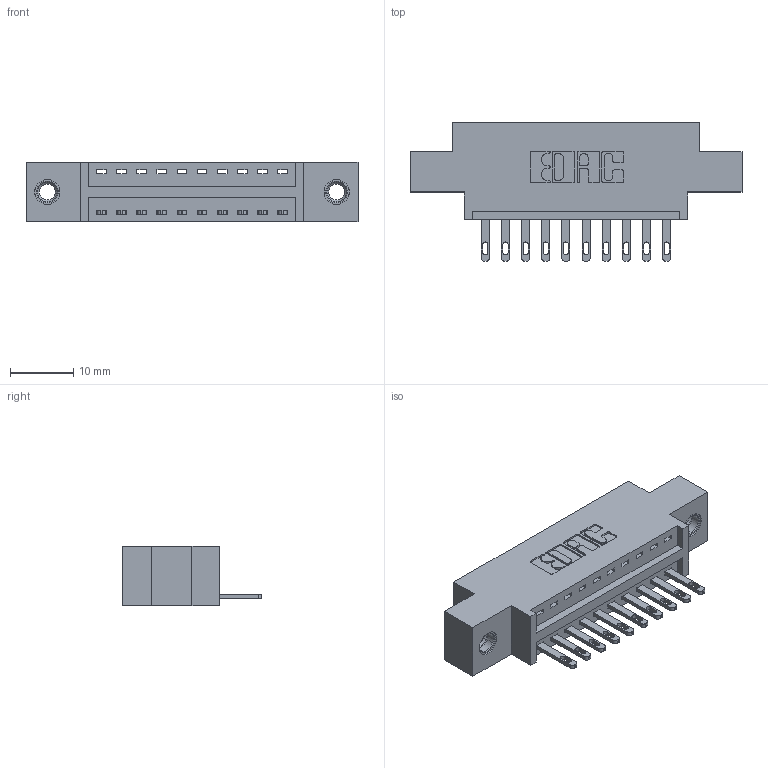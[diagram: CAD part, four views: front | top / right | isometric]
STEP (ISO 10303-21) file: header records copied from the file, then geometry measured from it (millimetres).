
FILE_DESCRIPTION (( 'STEP AP203' ), '1' );
FILE_NAME ('896-010-500-607.STEP', '2021-07-27T14:25:12', ( '' ), ( '' ), 'SwSTEP 2.0', 'SolidWorks 2020', '' );
FILE_SCHEMA (( 'CONFIG_CONTROL_DESIGN' ));
Length unit declared in the file: inch
Products named in the file (4): 846 Part_0.170 Offset - 0.156 Dia-TI; 345-292-001_345-293-100; 896-010-500-607; 345-250-001_345-250-005-103
Assembly tree (13 placements, depth 2):
  896-010-500-607
    846 Part_0.170 Offset - 0.156 Dia-TI
    345-292-001_345-293-100  x10
    345-250-001_345-250-005-103  x2
Bounding box: 52.32 x 21.84 x 9.4 mm (x, y, z)
Volume: 4626.2 mm3; surface area: 5655.1 mm2
Topology: 13 solids, 13 shells, 726 faces, 2157 edges, 1430 vertices
Faces by surface type: plane 452, cylinder 258, cone 12, torus 4
Entity records: 11762 total; most frequent: CARTESIAN_POINT 2009, ORIENTED_EDGE 1946, DIRECTION 1839, EDGE_CURVE 973, VECTOR 777, LINE 777, VERTEX_POINT 644, AXIS2_PLACEMENT_3D 531
